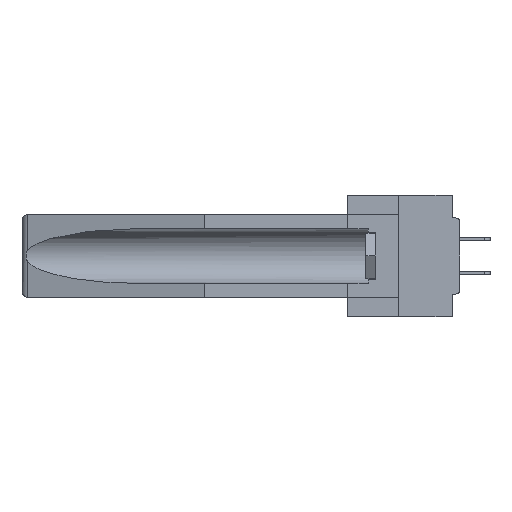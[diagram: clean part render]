
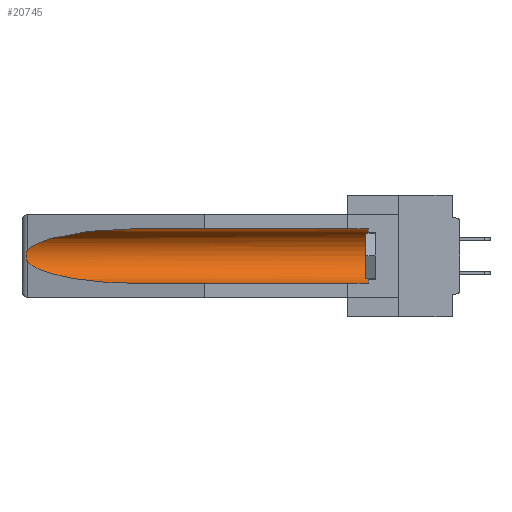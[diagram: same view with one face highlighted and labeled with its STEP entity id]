
A CAD part, left-side view. The second image highlights one B-rep face of the part: STEP entity #20745.
In plain terms, the highlighted cylindrical face has radius 2.857 mm (diameter 5.715 mm), a partial arc.
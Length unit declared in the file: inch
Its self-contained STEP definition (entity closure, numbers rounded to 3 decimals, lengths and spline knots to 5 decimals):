
#281 = EDGE_CURVE ( 'NONE', #12097, #22348, #26808, .T. ) ;
#422 = DIRECTION ( 'NONE',  ( 0., 1., 0. ) ) ;
#424 = CARTESIAN_POINT ( 'NONE',  ( 0.25451, 1.48313, -0.09465 ) ) ;
#466 = ORIENTED_EDGE ( 'NONE', *, *, #12628, .T. ) ;
#531 = CARTESIAN_POINT ( 'NONE',  ( 0.25451, 1.48313, -0.24835 ) ) ;
#1474 = VERTEX_POINT ( 'NONE', #21779 ) ;
#3177 = VECTOR ( 'NONE', #32531, 39.37008 ) ;
#3509 = VERTEX_POINT ( 'NONE', #33589 ) ;
#3580 = EDGE_CURVE ( 'NONE', #19313, #1474, #26531, .T. ) ;
#3897 = CARTESIAN_POINT ( 'NONE',  ( 0.155, 0.126, -0.1715 ) ) ;
#4833 = CARTESIAN_POINT ( 'NONE',  ( 0.155, 1.07973, -0.059 ) ) ;
#6081 = DIRECTION ( 'NONE',  ( 0., 0., 1. ) ) ;
#7196 = CYLINDRICAL_SURFACE ( 'NONE', #20967, 0.1125 ) ;
#7690 = B_SPLINE_CURVE_WITH_KNOTS ( 'NONE', 3,
 ( #8461, #14317, #8942, #14074, #25681, #31063, #11501, #25301, #33862, #22863 ),
 .UNSPECIFIED., .F., .F.,
 ( 4, 2, 2, 2, 4 ),
 ( 0., 0.00029, 0.00058, 0.00087, 0.00117 ),
 .UNSPECIFIED. ) ;
#8104 = EDGE_LOOP ( 'NONE', ( #20285, #30645, #30461, #27070, #466, #15201 ) ) ;
#8461 = CARTESIAN_POINT ( 'NONE',  ( 0.26537, 1.52718, -0.14972 ) ) ;
#8942 = CARTESIAN_POINT ( 'NONE',  ( 0.26654, 1.53092, -0.15636 ) ) ;
#10161 = CARTESIAN_POINT ( 'NONE',  ( 0.26537, 1.52718, -0.19328 ) ) ;
#11501 = CARTESIAN_POINT ( 'NONE',  ( 0.2673, 1.53269, -0.17917 ) ) ;
#11626 = CIRCLE ( 'NONE', #30392, 0.1125 ) ;
#11824 = CARTESIAN_POINT ( 'NONE',  ( 0.21114, 1.30732, -0.284 ) ) ;
#11947 = CARTESIAN_POINT ( 'NONE',  ( 0.155, 1.07973, -0.284 ) ) ;
#12097 = VERTEX_POINT ( 'NONE', #15333 ) ;
#12101 = DIRECTION ( 'NONE',  ( 0., -1., 0. ) ) ;
#12628 = EDGE_CURVE ( 'NONE', #12097, #3509, #11626, .T. ) ;
#13251 = DIRECTION ( 'NONE',  ( 0., 1., 0. ) ) ;
#14074 = CARTESIAN_POINT ( 'NONE',  ( 0.2673, 1.5327, -0.16383 ) ) ;
#14317 = CARTESIAN_POINT ( 'NONE',  ( 0.26597, 1.52961, -0.15275 ) ) ;
#15201 = ORIENTED_EDGE ( 'NONE', *, *, #21697, .T. ) ;
#15333 = CARTESIAN_POINT ( 'NONE',  ( 0.155, 0.126, -0.284 ) ) ;
#15404 = VERTEX_POINT ( 'NONE', #10161 ) ;
#17226 = CARTESIAN_POINT ( 'NONE',  ( 0.21114, 1.30732, -0.059 ) ) ;
#17704 = CARTESIAN_POINT ( 'NONE',  ( 0.155, 1.07973, -0.059 ) ) ;
#17732 = DIRECTION ( 'NONE',  ( 0., 0., 1. ) ) ;
#18375 = CARTESIAN_POINT ( 'NONE',  ( 0.155, -0.30754, -0.284 ) ) ;
#18387 = CARTESIAN_POINT ( 'NONE',  ( 0.155, -0.30754, -0.059 ) ) ;
#19313 = VERTEX_POINT ( 'NONE', #4833 ) ;
#20033 = CARTESIAN_POINT ( 'NONE',  ( 0.26537, 1.52718, -0.14972 ) ) ;
#20285 = ORIENTED_EDGE ( 'NONE', *, *, #3580, .T. ) ;
#20745 = ADVANCED_FACE ( 'NONE', ( #33430 ), #7196, .F. ) ;
#20967 = AXIS2_PLACEMENT_3D ( 'NONE', #22830, #422, #6081 ) ;
#21697 = EDGE_CURVE ( 'NONE', #3509, #19313, #33776, .T. ) ;
#21779 = CARTESIAN_POINT ( 'NONE',  ( 0.26537, 1.52718, -0.14972 ) ) ;
#22348 = VERTEX_POINT ( 'NONE', #23379 ) ;
#22830 = CARTESIAN_POINT ( 'NONE',  ( 0.155, -0.30754, -0.1715 ) ) ;
#22863 = CARTESIAN_POINT ( 'NONE',  ( 0.26537, 1.52718, -0.19328 ) ) ;
#22878 = EDGE_CURVE ( 'NONE', #1474, #15404, #7690, .T. ) ;
#23379 = CARTESIAN_POINT ( 'NONE',  ( 0.155, 1.07973, -0.284 ) ) ;
#25301 = CARTESIAN_POINT ( 'NONE',  ( 0.26655, 1.53094, -0.18657 ) ) ;
#25608 =( BOUNDED_CURVE ( )  B_SPLINE_CURVE ( 3, ( #28670, #531, #11824, #11947 ),
 .UNSPECIFIED., .F., .T. ) 
 B_SPLINE_CURVE_WITH_KNOTS ( ( 4, 4 ),
 ( 0.1948, 1.5708 ),
 .UNSPECIFIED. ) 
 CURVE ( )  GEOMETRIC_REPRESENTATION_ITEM ( )  RATIONAL_B_SPLINE_CURVE ( ( 1., 0.848, 0.848, 1. ) ) 
 REPRESENTATION_ITEM ( '' )  );
#25681 = CARTESIAN_POINT ( 'NONE',  ( 0.2675, 1.53308, -0.16763 ) ) ;
#26531 =( BOUNDED_CURVE ( )  B_SPLINE_CURVE ( 3, ( #17704, #17226, #424, #20033 ),
 .UNSPECIFIED., .F., .F. ) 
 B_SPLINE_CURVE_WITH_KNOTS ( ( 4, 4 ),
 ( 4.71239, 6.08839 ),
 .UNSPECIFIED. ) 
 CURVE ( )  GEOMETRIC_REPRESENTATION_ITEM ( )  RATIONAL_B_SPLINE_CURVE ( ( 1., 0.848, 0.848, 1. ) ) 
 REPRESENTATION_ITEM ( '' )  );
#26808 = LINE ( 'NONE', #18375, #3177 ) ;
#27070 = ORIENTED_EDGE ( 'NONE', *, *, #281, .F. ) ;
#28670 = CARTESIAN_POINT ( 'NONE',  ( 0.26537, 1.52718, -0.19328 ) ) ;
#30392 = AXIS2_PLACEMENT_3D ( 'NONE', #3897, #12101, #17732 ) ;
#30461 = ORIENTED_EDGE ( 'NONE', *, *, #32669, .T. ) ;
#30645 = ORIENTED_EDGE ( 'NONE', *, *, #22878, .T. ) ;
#31063 = CARTESIAN_POINT ( 'NONE',  ( 0.2675, 1.53308, -0.17534 ) ) ;
#32531 = DIRECTION ( 'NONE',  ( 0., 1., 0. ) ) ;
#32669 = EDGE_CURVE ( 'NONE', #15404, #22348, #25608, .T. ) ;
#33361 = VECTOR ( 'NONE', #13251, 39.37008 ) ;
#33430 = FACE_OUTER_BOUND ( 'NONE', #8104, .T. ) ;
#33589 = CARTESIAN_POINT ( 'NONE',  ( 0.155, 0.126, -0.059 ) ) ;
#33776 = LINE ( 'NONE', #18387, #33361 ) ;
#33862 = CARTESIAN_POINT ( 'NONE',  ( 0.26597, 1.5296, -0.19026 ) ) ;
